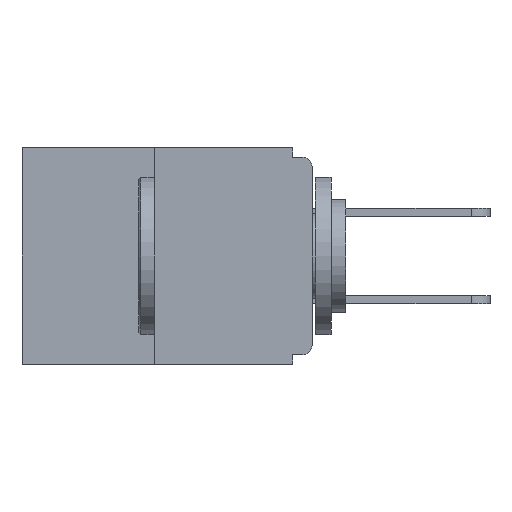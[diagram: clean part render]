
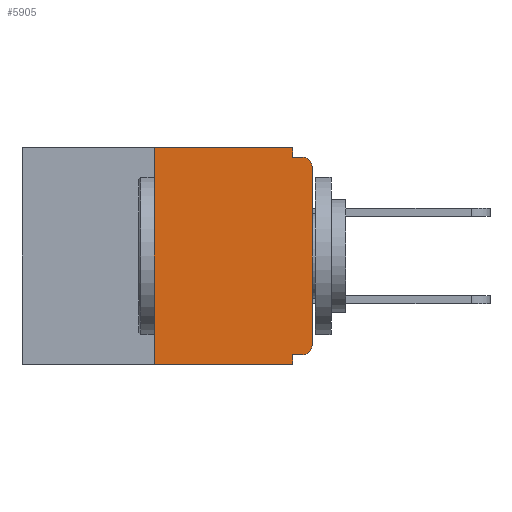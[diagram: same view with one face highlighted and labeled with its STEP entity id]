
A CAD part, left-side view. The second image highlights one B-rep face of the part: STEP entity #5905.
In plain terms, the highlighted planar face has unit normal (-1, 0, 0).
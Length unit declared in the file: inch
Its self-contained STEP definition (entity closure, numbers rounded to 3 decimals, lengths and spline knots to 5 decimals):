
#140 = EDGE_CURVE ( 'NONE', #3679, #8468, #13204, .T. ) ;
#193 = CARTESIAN_POINT ( 'NONE',  ( 0., 0., -0.015 ) ) ;
#371 = VECTOR ( 'NONE', #3378, 39.37008 ) ;
#623 = DIRECTION ( 'NONE',  ( 0., 0., -1. ) ) ;
#926 = CIRCLE ( 'NONE', #19908, 0.015 ) ;
#1070 = LINE ( 'NONE', #10258, #14406 ) ;
#2011 = LINE ( 'NONE', #6658, #371 ) ;
#2354 = VERTEX_POINT ( 'NONE', #5045 ) ;
#2776 = ORIENTED_EDGE ( 'NONE', *, *, #6338, .F. ) ;
#3079 = AXIS2_PLACEMENT_3D ( 'NONE', #13590, #11618, #15422 ) ;
#3220 = VECTOR ( 'NONE', #18467, 39.37008 ) ;
#3337 = DIRECTION ( 'NONE',  ( 0., 0., -1. ) ) ;
#3378 = DIRECTION ( 'NONE',  ( 0., 0., 1. ) ) ;
#3679 = VERTEX_POINT ( 'NONE', #5496 ) ;
#3802 = CARTESIAN_POINT ( 'NONE',  ( 0., 0.015, -0.313 ) ) ;
#3938 = ORIENTED_EDGE ( 'NONE', *, *, #9955, .F. ) ;
#4009 = LINE ( 'NONE', #13751, #11592 ) ;
#4143 = CARTESIAN_POINT ( 'NONE',  ( 0., 0.015, -0.03 ) ) ;
#4748 = VERTEX_POINT ( 'NONE', #17141 ) ;
#4942 = PLANE ( 'NONE',  #3079 ) ;
#5045 = CARTESIAN_POINT ( 'NONE',  ( 0., 0.031, -0.328 ) ) ;
#5365 = EDGE_CURVE ( 'NONE', #21385, #8072, #17113, .T. ) ;
#5496 = CARTESIAN_POINT ( 'NONE',  ( 0., 0.031, -0.015 ) ) ;
#5677 = DIRECTION ( 'NONE',  ( 0., -1., 0. ) ) ;
#5692 = CARTESIAN_POINT ( 'NONE',  ( 0., 0.25, 0. ) ) ;
#5905 = ADVANCED_FACE ( 'NONE', ( #8911 ), #4942, .F. ) ;
#6231 = ORIENTED_EDGE ( 'NONE', *, *, #11970, .T. ) ;
#6271 = VERTEX_POINT ( 'NONE', #11995 ) ;
#6338 = EDGE_CURVE ( 'NONE', #4748, #2354, #4009, .T. ) ;
#6658 = CARTESIAN_POINT ( 'NONE',  ( 0., 0., 0. ) ) ;
#6748 = DIRECTION ( 'NONE',  ( 0., -1., 0. ) ) ;
#7916 = DIRECTION ( 'NONE',  ( -1., 0., 0. ) ) ;
#7961 = VECTOR ( 'NONE', #19257, 39.37008 ) ;
#8057 = LINE ( 'NONE', #18848, #15130 ) ;
#8072 = VERTEX_POINT ( 'NONE', #21750 ) ;
#8468 = VERTEX_POINT ( 'NONE', #18486 ) ;
#8482 = LINE ( 'NONE', #17601, #7961 ) ;
#8661 = ORIENTED_EDGE ( 'NONE', *, *, #140, .F. ) ;
#8911 = FACE_OUTER_BOUND ( 'NONE', #17834, .T. ) ;
#9656 = CIRCLE ( 'NONE', #17967, 0.015 ) ;
#9955 = EDGE_CURVE ( 'NONE', #13693, #21385, #8482, .T. ) ;
#10258 = CARTESIAN_POINT ( 'NONE',  ( 0., 0.46, -0.343 ) ) ;
#10788 = DIRECTION ( 'NONE',  ( 0., 0., -1. ) ) ;
#11592 = VECTOR ( 'NONE', #20521, 39.37008 ) ;
#11618 = DIRECTION ( 'NONE',  ( 1., 0., 0. ) ) ;
#11746 = ORIENTED_EDGE ( 'NONE', *, *, #18033, .F. ) ;
#11970 = EDGE_CURVE ( 'NONE', #13693, #19267, #1070, .T. ) ;
#11995 = CARTESIAN_POINT ( 'NONE',  ( 0., 0., -0.313 ) ) ;
#13204 = LINE ( 'NONE', #193, #19174 ) ;
#13315 = VERTEX_POINT ( 'NONE', #16466 ) ;
#13590 = CARTESIAN_POINT ( 'NONE',  ( 0., 0.46, 0. ) ) ;
#13693 = VERTEX_POINT ( 'NONE', #14755 ) ;
#13751 = CARTESIAN_POINT ( 'NONE',  ( 0., 0., -0.328 ) ) ;
#14406 = VECTOR ( 'NONE', #6748, 39.37008 ) ;
#14755 = CARTESIAN_POINT ( 'NONE',  ( 0., 0.25, -0.343 ) ) ;
#14826 = CARTESIAN_POINT ( 'NONE',  ( 0., 0.46, 0. ) ) ;
#14912 = ORIENTED_EDGE ( 'NONE', *, *, #18117, .T. ) ;
#15130 = VECTOR ( 'NONE', #3337, 39.37008 ) ;
#15422 = DIRECTION ( 'NONE',  ( 0., 0., -1. ) ) ;
#15484 = VECTOR ( 'NONE', #623, 39.37008 ) ;
#16466 = CARTESIAN_POINT ( 'NONE',  ( 0., 0., -0.03 ) ) ;
#16654 = ORIENTED_EDGE ( 'NONE', *, *, #16710, .F. ) ;
#16710 = EDGE_CURVE ( 'NONE', #8072, #3679, #21199, .T. ) ;
#17113 = LINE ( 'NONE', #14826, #3220 ) ;
#17141 = CARTESIAN_POINT ( 'NONE',  ( 0., 0.015, -0.328 ) ) ;
#17601 = CARTESIAN_POINT ( 'NONE',  ( 0., 0.25, 0. ) ) ;
#17834 = EDGE_LOOP ( 'NONE', ( #22107, #3938, #6231, #11746, #2776, #14912, #21897, #20001, #8661, #16654 ) ) ;
#17967 = AXIS2_PLACEMENT_3D ( 'NONE', #3802, #20961, #10788 ) ;
#18033 = EDGE_CURVE ( 'NONE', #2354, #19267, #8057, .T. ) ;
#18041 = CARTESIAN_POINT ( 'NONE',  ( 0., 0.031, 0. ) ) ;
#18117 = EDGE_CURVE ( 'NONE', #4748, #6271, #9656, .T. ) ;
#18467 = DIRECTION ( 'NONE',  ( 0., -1., 0. ) ) ;
#18486 = CARTESIAN_POINT ( 'NONE',  ( 0., 0.015, -0.015 ) ) ;
#18848 = CARTESIAN_POINT ( 'NONE',  ( 0., 0.031, -0.343 ) ) ;
#19174 = VECTOR ( 'NONE', #5677, 39.37008 ) ;
#19257 = DIRECTION ( 'NONE',  ( 0., 0., 1. ) ) ;
#19267 = VERTEX_POINT ( 'NONE', #21502 ) ;
#19908 = AXIS2_PLACEMENT_3D ( 'NONE', #4143, #7916, #21543 ) ;
#20001 = ORIENTED_EDGE ( 'NONE', *, *, #20373, .T. ) ;
#20281 = EDGE_CURVE ( 'NONE', #6271, #13315, #2011, .T. ) ;
#20373 = EDGE_CURVE ( 'NONE', #13315, #8468, #926, .T. ) ;
#20521 = DIRECTION ( 'NONE',  ( 0., 1., 0. ) ) ;
#20961 = DIRECTION ( 'NONE',  ( -1., 0., 0. ) ) ;
#21199 = LINE ( 'NONE', #18041, #15484 ) ;
#21385 = VERTEX_POINT ( 'NONE', #5692 ) ;
#21502 = CARTESIAN_POINT ( 'NONE',  ( 0., 0.031, -0.343 ) ) ;
#21543 = DIRECTION ( 'NONE',  ( 0., 0., -1. ) ) ;
#21750 = CARTESIAN_POINT ( 'NONE',  ( 0., 0.031, 0. ) ) ;
#21897 = ORIENTED_EDGE ( 'NONE', *, *, #20281, .T. ) ;
#22107 = ORIENTED_EDGE ( 'NONE', *, *, #5365, .F. ) ;
